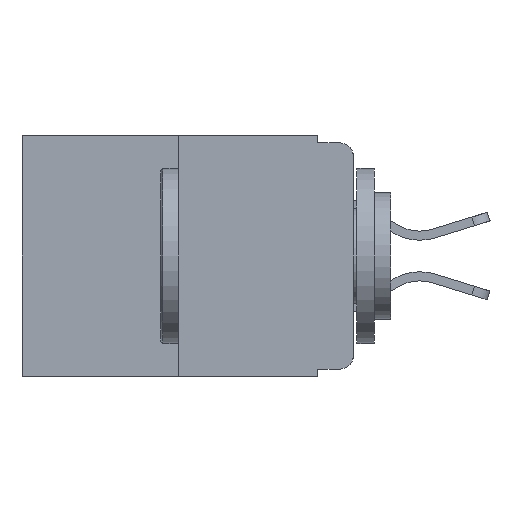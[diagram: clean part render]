
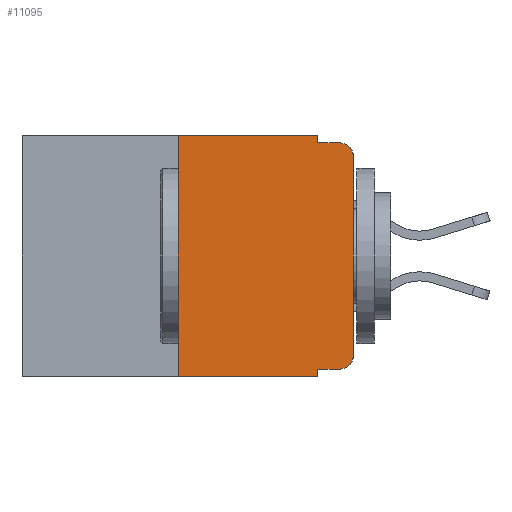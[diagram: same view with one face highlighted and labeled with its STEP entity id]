
A CAD part, left-side view. The second image highlights one B-rep face of the part: STEP entity #11095.
In plain terms, the highlighted planar face has unit normal (-1, 0, 0).
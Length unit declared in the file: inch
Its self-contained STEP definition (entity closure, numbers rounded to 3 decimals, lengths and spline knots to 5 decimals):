
#80 = AXIS2_PLACEMENT_3D ( 'NONE', #390, #386, #10169 ) ;
#386 = DIRECTION ( 'NONE',  ( -1., 0., 0. ) ) ;
#390 = CARTESIAN_POINT ( 'NONE',  ( 0., 0.02, -0.03 ) ) ;
#565 = ORIENTED_EDGE ( 'NONE', *, *, #2850, .T. ) ;
#621 = VECTOR ( 'NONE', #6896, 39.37008 ) ;
#637 = EDGE_CURVE ( 'NONE', #9617, #15476, #19478, .T. ) ;
#676 = ORIENTED_EDGE ( 'NONE', *, *, #1777, .T. ) ;
#845 = AXIS2_PLACEMENT_3D ( 'NONE', #13351, #3824, #14922 ) ;
#1002 = CARTESIAN_POINT ( 'NONE',  ( 0., 0.02, -0.01 ) ) ;
#1100 = ORIENTED_EDGE ( 'NONE', *, *, #637, .F. ) ;
#1149 = LINE ( 'NONE', #6862, #621 ) ;
#1341 = CARTESIAN_POINT ( 'NONE',  ( 0., 0.25, 0. ) ) ;
#1483 = ORIENTED_EDGE ( 'NONE', *, *, #20074, .F. ) ;
#1496 = VECTOR ( 'NONE', #13828, 39.37008 ) ;
#1527 = DIRECTION ( 'NONE',  ( 0., -1., 0. ) ) ;
#1611 = ORIENTED_EDGE ( 'NONE', *, *, #10208, .F. ) ;
#1649 = ORIENTED_EDGE ( 'NONE', *, *, #19051, .F. ) ;
#1737 = VECTOR ( 'NONE', #1527, 39.37008 ) ;
#1777 = EDGE_CURVE ( 'NONE', #5645, #15476, #8502, .T. ) ;
#1857 = CARTESIAN_POINT ( 'NONE',  ( 0., 0., -0.313 ) ) ;
#2327 = EDGE_LOOP ( 'NONE', ( #565, #676, #1100, #1483, #1611, #1649, #5372, #8541, #12460, #13386 ) ) ;
#2455 = CARTESIAN_POINT ( 'NONE',  ( 0., 0.051, -0.333 ) ) ;
#2850 = EDGE_CURVE ( 'NONE', #3126, #5645, #1149, .T. ) ;
#3126 = VERTEX_POINT ( 'NONE', #1857 ) ;
#3444 = VERTEX_POINT ( 'NONE', #13415 ) ;
#3604 = VERTEX_POINT ( 'NONE', #1341 ) ;
#3734 = LINE ( 'NONE', #2455, #16362 ) ;
#3824 = DIRECTION ( 'NONE',  ( 1., 0., 0. ) ) ;
#4293 = VERTEX_POINT ( 'NONE', #4300 ) ;
#4300 = CARTESIAN_POINT ( 'NONE',  ( 0., 0.051, -0.343 ) ) ;
#5372 = ORIENTED_EDGE ( 'NONE', *, *, #8905, .T. ) ;
#5595 = DIRECTION ( 'NONE',  ( -1., 0., 0. ) ) ;
#5645 = VERTEX_POINT ( 'NONE', #11751 ) ;
#6183 = LINE ( 'NONE', #20287, #14132 ) ;
#6862 = CARTESIAN_POINT ( 'NONE',  ( 0., 0., 0. ) ) ;
#6896 = DIRECTION ( 'NONE',  ( 0., 0., 1. ) ) ;
#7060 = CARTESIAN_POINT ( 'NONE',  ( 0., 0.051, 0. ) ) ;
#8059 = DIRECTION ( 'NONE',  ( 0., 0., 1. ) ) ;
#8502 = CIRCLE ( 'NONE', #80, 0.02 ) ;
#8541 = ORIENTED_EDGE ( 'NONE', *, *, #18038, .F. ) ;
#8572 = LINE ( 'NONE', #7060, #19997 ) ;
#8674 = DIRECTION ( 'NONE',  ( 0., 0., -1. ) ) ;
#8838 = CARTESIAN_POINT ( 'NONE',  ( 0., 0.02, -0.333 ) ) ;
#8905 = EDGE_CURVE ( 'NONE', #11305, #4293, #13709, .T. ) ;
#9079 = CARTESIAN_POINT ( 'NONE',  ( 0., 0.473, -0.343 ) ) ;
#9095 = FACE_OUTER_BOUND ( 'NONE', #2327, .T. ) ;
#9501 = CARTESIAN_POINT ( 'NONE',  ( 0., 0.473, 0. ) ) ;
#9617 = VERTEX_POINT ( 'NONE', #17526 ) ;
#10169 = DIRECTION ( 'NONE',  ( 0., 0., -1. ) ) ;
#10208 = EDGE_CURVE ( 'NONE', #3604, #17740, #10716, .T. ) ;
#10523 = CIRCLE ( 'NONE', #17910, 0.02 ) ;
#10561 = VERTEX_POINT ( 'NONE', #8838 ) ;
#10716 = LINE ( 'NONE', #9501, #1737 ) ;
#10997 = DIRECTION ( 'NONE',  ( 0., 0., -1. ) ) ;
#11095 = ADVANCED_FACE ( 'NONE', ( #9095 ), #17953, .F. ) ;
#11305 = VERTEX_POINT ( 'NONE', #15390 ) ;
#11718 = VECTOR ( 'NONE', #16261, 39.37008 ) ;
#11751 = CARTESIAN_POINT ( 'NONE',  ( 0., 0., -0.03 ) ) ;
#12460 = ORIENTED_EDGE ( 'NONE', *, *, #17023, .T. ) ;
#13351 = CARTESIAN_POINT ( 'NONE',  ( 0., 0.473, 0. ) ) ;
#13386 = ORIENTED_EDGE ( 'NONE', *, *, #15986, .T. ) ;
#13415 = CARTESIAN_POINT ( 'NONE',  ( 0., 0.051, -0.333 ) ) ;
#13459 = LINE ( 'NONE', #14335, #16624 ) ;
#13709 = LINE ( 'NONE', #9079, #1496 ) ;
#13828 = DIRECTION ( 'NONE',  ( 0., -1., 0. ) ) ;
#14132 = VECTOR ( 'NONE', #10997, 39.37008 ) ;
#14184 = CARTESIAN_POINT ( 'NONE',  ( 0., 0.051, 0. ) ) ;
#14335 = CARTESIAN_POINT ( 'NONE',  ( 0., 0.25, 0. ) ) ;
#14922 = DIRECTION ( 'NONE',  ( 0., 0., -1. ) ) ;
#15114 = CARTESIAN_POINT ( 'NONE',  ( 0., 0.02, -0.313 ) ) ;
#15390 = CARTESIAN_POINT ( 'NONE',  ( 0., 0.25, -0.343 ) ) ;
#15476 = VERTEX_POINT ( 'NONE', #1002 ) ;
#15986 = EDGE_CURVE ( 'NONE', #10561, #3126, #10523, .T. ) ;
#16261 = DIRECTION ( 'NONE',  ( 0., -1., 0. ) ) ;
#16362 = VECTOR ( 'NONE', #16710, 39.37008 ) ;
#16624 = VECTOR ( 'NONE', #8059, 39.37008 ) ;
#16678 = DIRECTION ( 'NONE',  ( 0., 0., -1. ) ) ;
#16710 = DIRECTION ( 'NONE',  ( 0., -1., 0. ) ) ;
#17023 = EDGE_CURVE ( 'NONE', #3444, #10561, #3734, .T. ) ;
#17526 = CARTESIAN_POINT ( 'NONE',  ( 0., 0.051, -0.01 ) ) ;
#17740 = VERTEX_POINT ( 'NONE', #14184 ) ;
#17910 = AXIS2_PLACEMENT_3D ( 'NONE', #15114, #5595, #16678 ) ;
#17953 = PLANE ( 'NONE',  #845 ) ;
#18038 = EDGE_CURVE ( 'NONE', #3444, #4293, #8572, .T. ) ;
#18662 = CARTESIAN_POINT ( 'NONE',  ( 0., 0.051, -0.01 ) ) ;
#19051 = EDGE_CURVE ( 'NONE', #11305, #3604, #13459, .T. ) ;
#19478 = LINE ( 'NONE', #18662, #11718 ) ;
#19997 = VECTOR ( 'NONE', #8674, 39.37008 ) ;
#20074 = EDGE_CURVE ( 'NONE', #17740, #9617, #6183, .T. ) ;
#20287 = CARTESIAN_POINT ( 'NONE',  ( 0., 0.051, 0. ) ) ;
